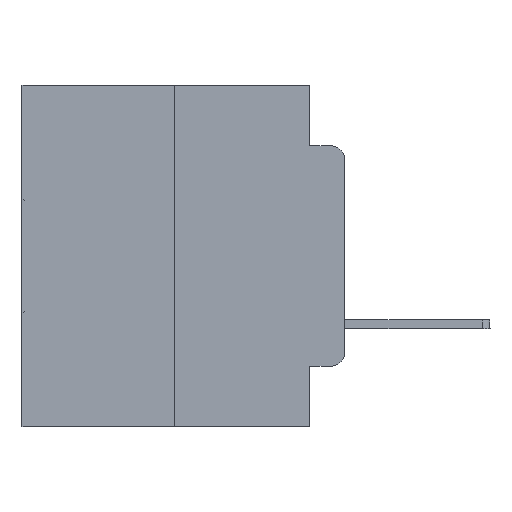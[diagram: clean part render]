
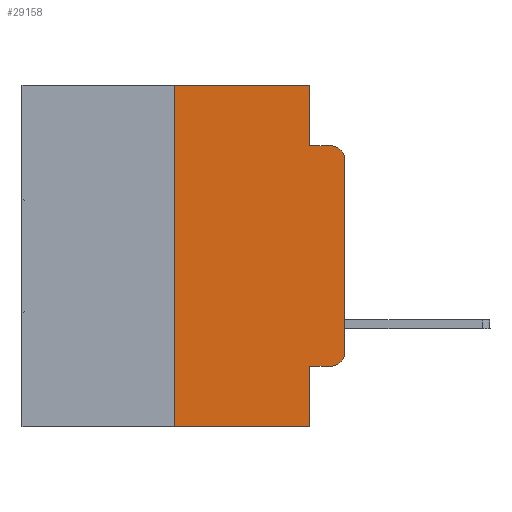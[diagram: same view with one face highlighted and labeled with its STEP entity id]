
A CAD part, left-side view. The second image highlights one B-rep face of the part: STEP entity #29158.
In plain terms, the highlighted planar face has unit normal (-1, 0, 0).
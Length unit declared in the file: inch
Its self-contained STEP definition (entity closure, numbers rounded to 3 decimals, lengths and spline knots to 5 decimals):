
#211 = VERTEX_POINT ( 'NONE', #19229 ) ;
#360 = AXIS2_PLACEMENT_3D ( 'NONE', #18951, #21268, #23648 ) ;
#644 = CARTESIAN_POINT ( 'NONE',  ( 0., 0.473, 0. ) ) ;
#1025 = CARTESIAN_POINT ( 'NONE',  ( 0., 0.473, -0.5 ) ) ;
#1255 = DIRECTION ( 'NONE',  ( 0., 0., -1. ) ) ;
#1281 = LINE ( 'NONE', #1025, #10862 ) ;
#1310 = CARTESIAN_POINT ( 'NONE',  ( 0., 0.25, 0. ) ) ;
#1869 = AXIS2_PLACEMENT_3D ( 'NONE', #644, #27188, #15489 ) ;
#2276 = VECTOR ( 'NONE', #29405, 39.37008 ) ;
#2694 = VERTEX_POINT ( 'NONE', #7938 ) ;
#2769 = CARTESIAN_POINT ( 'NONE',  ( 0., 0.473, 0. ) ) ;
#2907 = VECTOR ( 'NONE', #15067, 39.37008 ) ;
#3172 = VERTEX_POINT ( 'NONE', #5849 ) ;
#3988 = VERTEX_POINT ( 'NONE', #21511 ) ;
#4030 = VERTEX_POINT ( 'NONE', #9807 ) ;
#4301 = EDGE_CURVE ( 'NONE', #211, #2694, #16386, .T. ) ;
#4478 = ORIENTED_EDGE ( 'NONE', *, *, #7336, .T. ) ;
#4809 = DIRECTION ( 'NONE',  ( 0., -1., 0. ) ) ;
#4970 = LINE ( 'NONE', #20268, #21878 ) ;
#5651 = EDGE_CURVE ( 'NONE', #26351, #4030, #14816, .T. ) ;
#5849 = CARTESIAN_POINT ( 'NONE',  ( 0., 0.02, -0.0885 ) ) ;
#5880 = CARTESIAN_POINT ( 'NONE',  ( 0., 0.051, -0.5 ) ) ;
#5999 = CARTESIAN_POINT ( 'NONE',  ( 0., 0.051, 0. ) ) ;
#6214 = DIRECTION ( 'NONE',  ( 0., 0., -1. ) ) ;
#6354 = CIRCLE ( 'NONE', #360, 0.02 ) ;
#7297 = ORIENTED_EDGE ( 'NONE', *, *, #21843, .F. ) ;
#7336 = EDGE_CURVE ( 'NONE', #2694, #12876, #21321, .T. ) ;
#7938 = CARTESIAN_POINT ( 'NONE',  ( 0., 0.02, -0.4115 ) ) ;
#8044 = CARTESIAN_POINT ( 'NONE',  ( 0., 0., -0.3915 ) ) ;
#8405 = EDGE_CURVE ( 'NONE', #30339, #3172, #10298, .T. ) ;
#9627 = ORIENTED_EDGE ( 'NONE', *, *, #24521, .F. ) ;
#9807 = CARTESIAN_POINT ( 'NONE',  ( 0., 0.25, 0. ) ) ;
#9925 = ORIENTED_EDGE ( 'NONE', *, *, #16661, .T. ) ;
#10298 = LINE ( 'NONE', #17026, #2907 ) ;
#10425 = LINE ( 'NONE', #5999, #22189 ) ;
#10862 = VECTOR ( 'NONE', #22300, 39.37008 ) ;
#11451 = ORIENTED_EDGE ( 'NONE', *, *, #8405, .F. ) ;
#11524 = ORIENTED_EDGE ( 'NONE', *, *, #4301, .T. ) ;
#12071 = EDGE_LOOP ( 'NONE', ( #9925, #24473, #11451, #7297, #9627, #22205, #16142, #13050, #11524, #4478 ) ) ;
#12426 = EDGE_CURVE ( 'NONE', #211, #21131, #10425, .T. ) ;
#12693 = CARTESIAN_POINT ( 'NONE',  ( 0., 0., 0. ) ) ;
#12812 = PLANE ( 'NONE',  #1869 ) ;
#12876 = VERTEX_POINT ( 'NONE', #8044 ) ;
#13050 = ORIENTED_EDGE ( 'NONE', *, *, #12426, .F. ) ;
#13720 = VECTOR ( 'NONE', #19256, 39.37008 ) ;
#13915 = AXIS2_PLACEMENT_3D ( 'NONE', #22637, #15392, #1255 ) ;
#14816 = LINE ( 'NONE', #1310, #2276 ) ;
#15067 = DIRECTION ( 'NONE',  ( 0., -1., 0. ) ) ;
#15392 = DIRECTION ( 'NONE',  ( -1., 0., 0. ) ) ;
#15486 = CARTESIAN_POINT ( 'NONE',  ( 0., 0.25, -0.5 ) ) ;
#15489 = DIRECTION ( 'NONE',  ( 0., 0., -1. ) ) ;
#15596 = LINE ( 'NONE', #12693, #19575 ) ;
#16142 = ORIENTED_EDGE ( 'NONE', *, *, #27831, .T. ) ;
#16386 = LINE ( 'NONE', #25287, #28165 ) ;
#16661 = EDGE_CURVE ( 'NONE', #12876, #30307, #15596, .T. ) ;
#17026 = CARTESIAN_POINT ( 'NONE',  ( 0., 0.051, -0.0885 ) ) ;
#18951 = CARTESIAN_POINT ( 'NONE',  ( 0., 0.02, -0.1085 ) ) ;
#19229 = CARTESIAN_POINT ( 'NONE',  ( 0., 0.051, -0.4115 ) ) ;
#19256 = DIRECTION ( 'NONE',  ( 0., -1., 0. ) ) ;
#19575 = VECTOR ( 'NONE', #21980, 39.37008 ) ;
#20268 = CARTESIAN_POINT ( 'NONE',  ( 0., 0.051, 0. ) ) ;
#21131 = VERTEX_POINT ( 'NONE', #5880 ) ;
#21268 = DIRECTION ( 'NONE',  ( -1., 0., 0. ) ) ;
#21321 = CIRCLE ( 'NONE', #13915, 0.02 ) ;
#21511 = CARTESIAN_POINT ( 'NONE',  ( 0., 0.051, 0. ) ) ;
#21843 = EDGE_CURVE ( 'NONE', #3988, #30339, #4970, .T. ) ;
#21878 = VECTOR ( 'NONE', #25437, 39.37008 ) ;
#21980 = DIRECTION ( 'NONE',  ( 0., 0., 1. ) ) ;
#22189 = VECTOR ( 'NONE', #6214, 39.37008 ) ;
#22205 = ORIENTED_EDGE ( 'NONE', *, *, #5651, .F. ) ;
#22300 = DIRECTION ( 'NONE',  ( 0., -1., 0. ) ) ;
#22637 = CARTESIAN_POINT ( 'NONE',  ( 0., 0.02, -0.3915 ) ) ;
#23403 = EDGE_CURVE ( 'NONE', #30307, #3172, #6354, .T. ) ;
#23648 = DIRECTION ( 'NONE',  ( 0., 0., -1. ) ) ;
#23971 = CARTESIAN_POINT ( 'NONE',  ( 0., 0., -0.1085 ) ) ;
#23980 = FACE_OUTER_BOUND ( 'NONE', #12071, .T. ) ;
#24473 = ORIENTED_EDGE ( 'NONE', *, *, #23403, .T. ) ;
#24521 = EDGE_CURVE ( 'NONE', #4030, #3988, #26191, .T. ) ;
#25287 = CARTESIAN_POINT ( 'NONE',  ( 0., 0.051, -0.4115 ) ) ;
#25437 = DIRECTION ( 'NONE',  ( 0., 0., -1. ) ) ;
#26191 = LINE ( 'NONE', #2769, #13720 ) ;
#26351 = VERTEX_POINT ( 'NONE', #15486 ) ;
#27188 = DIRECTION ( 'NONE',  ( 1., 0., 0. ) ) ;
#27831 = EDGE_CURVE ( 'NONE', #26351, #21131, #1281, .T. ) ;
#28165 = VECTOR ( 'NONE', #4809, 39.37008 ) ;
#28625 = CARTESIAN_POINT ( 'NONE',  ( 0., 0.051, -0.0885 ) ) ;
#29158 = ADVANCED_FACE ( 'NONE', ( #23980 ), #12812, .F. ) ;
#29405 = DIRECTION ( 'NONE',  ( 0., 0., 1. ) ) ;
#30307 = VERTEX_POINT ( 'NONE', #23971 ) ;
#30339 = VERTEX_POINT ( 'NONE', #28625 ) ;
